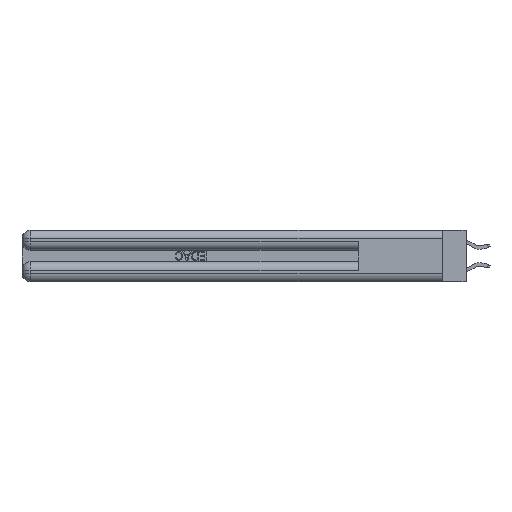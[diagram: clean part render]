
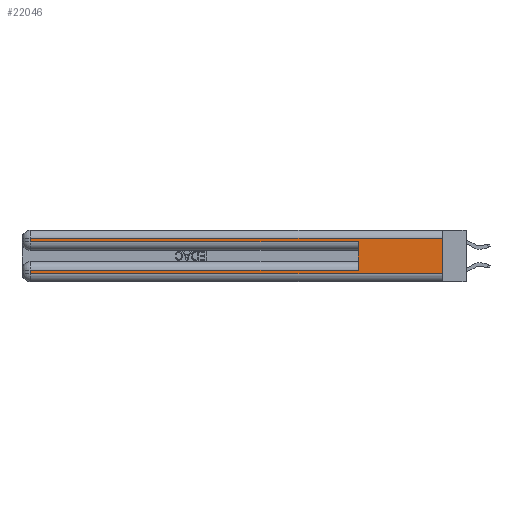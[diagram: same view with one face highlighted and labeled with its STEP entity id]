
A CAD part, left-side view. The second image highlights one B-rep face of the part: STEP entity #22046.
In plain terms, the highlighted planar face has unit normal (-1, 0, 0).
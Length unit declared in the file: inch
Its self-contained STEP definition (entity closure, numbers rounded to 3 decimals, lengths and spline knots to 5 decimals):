
#236 = ORIENTED_EDGE ( 'NONE', *, *, #13324, .F. ) ;
#279 = DIRECTION ( 'NONE',  ( 0., -1., 0. ) ) ;
#1214 = VECTOR ( 'NONE', #279, 39.37008 ) ;
#1601 = DIRECTION ( 'NONE',  ( 0., 0., -1. ) ) ;
#2013 = DIRECTION ( 'NONE',  ( 0., 0., -1. ) ) ;
#2499 = CARTESIAN_POINT ( 'NONE',  ( 0., 2.94, 0.285 ) ) ;
#3626 = EDGE_CURVE ( 'NONE', #16720, #28086, #23869, .T. ) ;
#3994 = LINE ( 'NONE', #28935, #33363 ) ;
#3999 = CARTESIAN_POINT ( 'NONE',  ( 0., 0., 0.06 ) ) ;
#4806 = VERTEX_POINT ( 'NONE', #22656 ) ;
#6740 = LINE ( 'NONE', #29322, #30924 ) ;
#7464 = ORIENTED_EDGE ( 'NONE', *, *, #32704, .F. ) ;
#7610 = VECTOR ( 'NONE', #15561, 39.37008 ) ;
#9796 = VECTOR ( 'NONE', #22721, 39.37008 ) ;
#9946 = CARTESIAN_POINT ( 'NONE',  ( 0., 0., 0.31 ) ) ;
#10815 = ORIENTED_EDGE ( 'NONE', *, *, #30358, .T. ) ;
#11027 = ORIENTED_EDGE ( 'NONE', *, *, #33390, .T. ) ;
#11478 = CARTESIAN_POINT ( 'NONE',  ( 0., 0., 0.37 ) ) ;
#11586 = VERTEX_POINT ( 'NONE', #14254 ) ;
#11638 = EDGE_CURVE ( 'NONE', #22913, #11799, #14778, .T. ) ;
#11690 = VERTEX_POINT ( 'NONE', #20076 ) ;
#11794 = LINE ( 'NONE', #28061, #1214 ) ;
#11799 = VERTEX_POINT ( 'NONE', #16514 ) ;
#12464 = CARTESIAN_POINT ( 'NONE',  ( 0., 2.94, 0.37 ) ) ;
#12919 = CARTESIAN_POINT ( 'NONE',  ( 0., 2.94, 0.06 ) ) ;
#13324 = EDGE_CURVE ( 'NONE', #4806, #11586, #29178, .T. ) ;
#13670 = VECTOR ( 'NONE', #32368, 39.37008 ) ;
#13960 = CARTESIAN_POINT ( 'NONE',  ( 0., 0., 0.37 ) ) ;
#14254 = CARTESIAN_POINT ( 'NONE',  ( 0., 0.6, 0.285 ) ) ;
#14778 = LINE ( 'NONE', #3999, #9796 ) ;
#15137 = DIRECTION ( 'NONE',  ( 0., 1., 0. ) ) ;
#15273 = VECTOR ( 'NONE', #18561, 39.37008 ) ;
#15561 = DIRECTION ( 'NONE',  ( 0., 0., 1. ) ) ;
#16514 = CARTESIAN_POINT ( 'NONE',  ( 0., 0., 0.06 ) ) ;
#16533 = VECTOR ( 'NONE', #2013, 39.37008 ) ;
#16720 = VERTEX_POINT ( 'NONE', #32106 ) ;
#16885 = AXIS2_PLACEMENT_3D ( 'NONE', #11478, #22412, #30922 ) ;
#16947 = PLANE ( 'NONE',  #16885 ) ;
#18019 = ORIENTED_EDGE ( 'NONE', *, *, #30159, .T. ) ;
#18310 = CARTESIAN_POINT ( 'NONE',  ( 0., 2.94, 0.31 ) ) ;
#18561 = DIRECTION ( 'NONE',  ( 0., 1., 0. ) ) ;
#19209 = VERTEX_POINT ( 'NONE', #2499 ) ;
#20076 = CARTESIAN_POINT ( 'NONE',  ( 0., 2.94, 0.085 ) ) ;
#20744 = LINE ( 'NONE', #12464, #16533 ) ;
#20754 = ORIENTED_EDGE ( 'NONE', *, *, #3626, .T. ) ;
#21658 = EDGE_LOOP ( 'NONE', ( #7464, #20754, #24857, #18019, #236, #10815, #11027, #34237 ) ) ;
#22046 = ADVANCED_FACE ( 'NONE', ( #25250 ), #16947, .F. ) ;
#22076 = LINE ( 'NONE', #13960, #13670 ) ;
#22412 = DIRECTION ( 'NONE',  ( 1., 0., 0. ) ) ;
#22656 = CARTESIAN_POINT ( 'NONE',  ( 0., 0.6, 0.085 ) ) ;
#22721 = DIRECTION ( 'NONE',  ( 0., -1., 0. ) ) ;
#22913 = VERTEX_POINT ( 'NONE', #12919 ) ;
#23869 = LINE ( 'NONE', #9946, #15273 ) ;
#24720 = EDGE_CURVE ( 'NONE', #28086, #19209, #6740, .T. ) ;
#24857 = ORIENTED_EDGE ( 'NONE', *, *, #24720, .T. ) ;
#25250 = FACE_OUTER_BOUND ( 'NONE', #21658, .T. ) ;
#28061 = CARTESIAN_POINT ( 'NONE',  ( 0., 0., 0.285 ) ) ;
#28086 = VERTEX_POINT ( 'NONE', #18310 ) ;
#28935 = CARTESIAN_POINT ( 'NONE',  ( 0., 0., 0.085 ) ) ;
#29178 = LINE ( 'NONE', #32353, #7610 ) ;
#29322 = CARTESIAN_POINT ( 'NONE',  ( 0., 2.94, 0.37 ) ) ;
#30159 = EDGE_CURVE ( 'NONE', #19209, #11586, #11794, .T. ) ;
#30358 = EDGE_CURVE ( 'NONE', #4806, #11690, #3994, .T. ) ;
#30922 = DIRECTION ( 'NONE',  ( 0., 0., -1. ) ) ;
#30924 = VECTOR ( 'NONE', #1601, 39.37008 ) ;
#32106 = CARTESIAN_POINT ( 'NONE',  ( 0., 0., 0.31 ) ) ;
#32353 = CARTESIAN_POINT ( 'NONE',  ( 0., 0.6, 0.145 ) ) ;
#32368 = DIRECTION ( 'NONE',  ( 0., 0., -1. ) ) ;
#32704 = EDGE_CURVE ( 'NONE', #16720, #11799, #22076, .T. ) ;
#33363 = VECTOR ( 'NONE', #15137, 39.37008 ) ;
#33390 = EDGE_CURVE ( 'NONE', #11690, #22913, #20744, .T. ) ;
#34237 = ORIENTED_EDGE ( 'NONE', *, *, #11638, .T. ) ;
